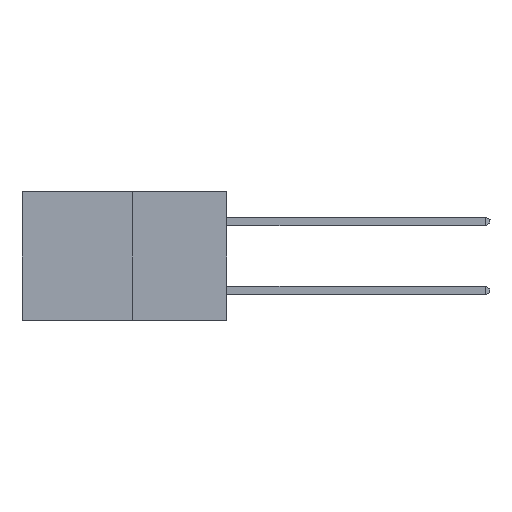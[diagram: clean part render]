
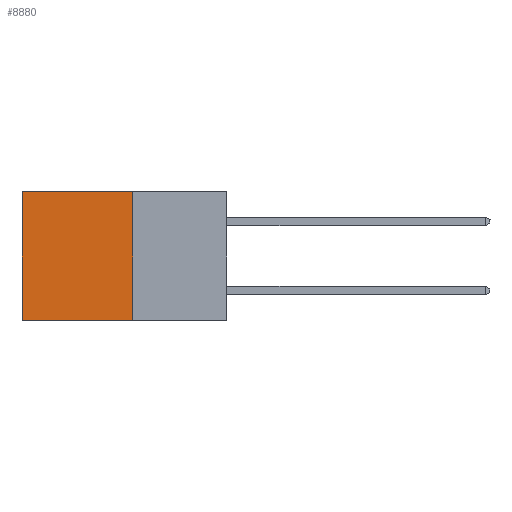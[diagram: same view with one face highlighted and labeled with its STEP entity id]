
A CAD part, left-side view. The second image highlights one B-rep face of the part: STEP entity #8880.
In plain terms, the highlighted planar face has unit normal (-1, 0, 0).
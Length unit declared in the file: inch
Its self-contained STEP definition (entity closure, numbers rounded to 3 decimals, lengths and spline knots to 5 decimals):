
#1539 = EDGE_CURVE ( 'NONE', #5875, #6523, #24439, .T. ) ;
#4206 = VECTOR ( 'NONE', #6321, 39.37008 ) ;
#4671 = LINE ( 'NONE', #15079, #17314 ) ;
#5875 = VERTEX_POINT ( 'NONE', #14318 ) ;
#6222 = VERTEX_POINT ( 'NONE', #20995 ) ;
#6321 = DIRECTION ( 'NONE',  ( 0., 1., 0. ) ) ;
#6357 = VERTEX_POINT ( 'NONE', #10599 ) ;
#6523 = VERTEX_POINT ( 'NONE', #29474 ) ;
#8017 = PLANE ( 'NONE',  #10173 ) ;
#8761 = DIRECTION ( 'NONE',  ( 0., 1., 0. ) ) ;
#8880 = ADVANCED_FACE ( 'NONE', ( #16376 ), #8017, .F. ) ;
#10173 = AXIS2_PLACEMENT_3D ( 'NONE', #18092, #10525, #28140 ) ;
#10525 = DIRECTION ( 'NONE',  ( 1., 0., 0. ) ) ;
#10599 = CARTESIAN_POINT ( 'NONE',  ( 0.277, 0.27, 0. ) ) ;
#13308 = ORIENTED_EDGE ( 'NONE', *, *, #1539, .T. ) ;
#13693 = ORIENTED_EDGE ( 'NONE', *, *, #13778, .T. ) ;
#13778 = EDGE_CURVE ( 'NONE', #6357, #5875, #24337, .T. ) ;
#14318 = CARTESIAN_POINT ( 'NONE',  ( 0.277, 0.59, 0. ) ) ;
#15079 = CARTESIAN_POINT ( 'NONE',  ( 0.277, 0.27, -0.37 ) ) ;
#15313 = VECTOR ( 'NONE', #8761, 39.37008 ) ;
#16376 = FACE_OUTER_BOUND ( 'NONE', #19027, .T. ) ;
#17314 = VECTOR ( 'NONE', #30114, 39.37008 ) ;
#17723 = VECTOR ( 'NONE', #24649, 39.37008 ) ;
#17776 = ORIENTED_EDGE ( 'NONE', *, *, #32348, .F. ) ;
#18092 = CARTESIAN_POINT ( 'NONE',  ( 0.277, 0.27, -0.37 ) ) ;
#18875 = CARTESIAN_POINT ( 'NONE',  ( 0.277, 0.27, -0.37 ) ) ;
#19027 = EDGE_LOOP ( 'NONE', ( #13308, #17776, #20018, #13693 ) ) ;
#20018 = ORIENTED_EDGE ( 'NONE', *, *, #32007, .F. ) ;
#20995 = CARTESIAN_POINT ( 'NONE',  ( 0.277, 0.27, -0.37 ) ) ;
#21292 = LINE ( 'NONE', #18875, #15313 ) ;
#21522 = CARTESIAN_POINT ( 'NONE',  ( 0.277, 0.27, 0. ) ) ;
#24337 = LINE ( 'NONE', #21522, #4206 ) ;
#24439 = LINE ( 'NONE', #26697, #17723 ) ;
#24649 = DIRECTION ( 'NONE',  ( 0., 0., -1. ) ) ;
#26697 = CARTESIAN_POINT ( 'NONE',  ( 0.277, 0.59, -0.37 ) ) ;
#28140 = DIRECTION ( 'NONE',  ( 0., 0., -1. ) ) ;
#29474 = CARTESIAN_POINT ( 'NONE',  ( 0.277, 0.59, -0.37 ) ) ;
#30114 = DIRECTION ( 'NONE',  ( 0., 0., -1. ) ) ;
#32007 = EDGE_CURVE ( 'NONE', #6357, #6222, #4671, .T. ) ;
#32348 = EDGE_CURVE ( 'NONE', #6222, #6523, #21292, .T. ) ;
